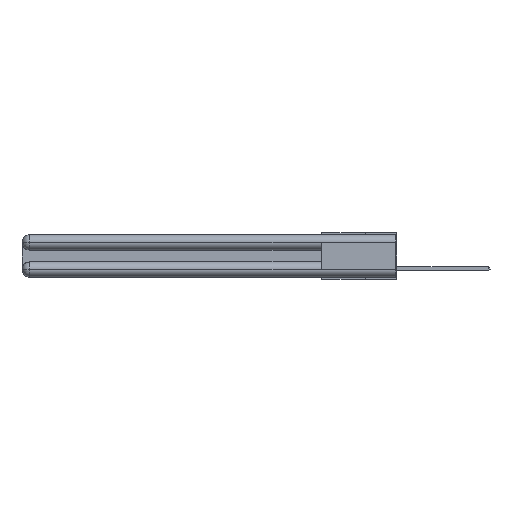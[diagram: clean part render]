
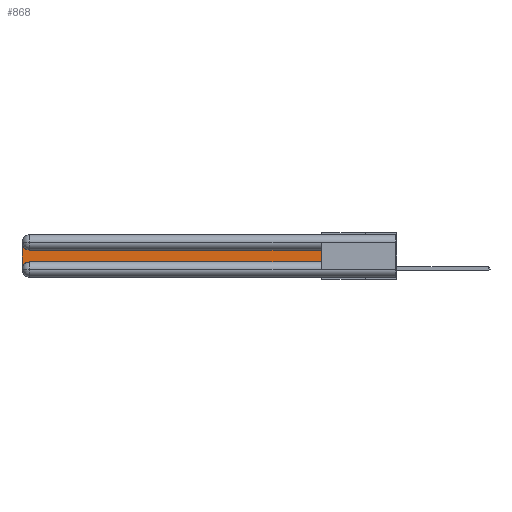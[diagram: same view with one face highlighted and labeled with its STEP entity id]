
A CAD part, left-side view. The second image highlights one B-rep face of the part: STEP entity #868.
In plain terms, the highlighted planar face has unit normal (-1, 0, 0).
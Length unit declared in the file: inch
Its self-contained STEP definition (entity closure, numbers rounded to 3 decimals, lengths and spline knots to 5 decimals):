
#131 = EDGE_CURVE ( 'NONE', #12326, #11056, #25993, .T. ) ;
#260 = PLANE ( 'NONE',  #14001 ) ;
#305 = DIRECTION ( 'NONE',  ( 1., 0., 0. ) ) ;
#825 = EDGE_CURVE ( 'NONE', #18323, #15972, #5601, .T. ) ;
#868 = ADVANCED_FACE ( 'NONE', ( #21508 ), #260, .F. ) ;
#1314 = CARTESIAN_POINT ( 'NONE',  ( 0.075, 3., -0.2175 ) ) ;
#3848 = ORIENTED_EDGE ( 'NONE', *, *, #825, .T. ) ;
#4190 = LINE ( 'NONE', #9751, #19255 ) ;
#5068 = LINE ( 'NONE', #8407, #24976 ) ;
#5601 = CIRCLE ( 'NONE', #16612, 0.06 ) ;
#8343 = LINE ( 'NONE', #31361, #13240 ) ;
#8407 = CARTESIAN_POINT ( 'NONE',  ( 0.075, 0.6, -0.2175 ) ) ;
#8570 = ORIENTED_EDGE ( 'NONE', *, *, #18665, .T. ) ;
#9751 = CARTESIAN_POINT ( 'NONE',  ( 0.075, 0.6, -0.2175 ) ) ;
#9907 = VECTOR ( 'NONE', #11904, 39.37008 ) ;
#10162 = DIRECTION ( 'NONE',  ( 0., 0., -1. ) ) ;
#11056 = VERTEX_POINT ( 'NONE', #21473 ) ;
#11326 = CARTESIAN_POINT ( 'NONE',  ( 0.075, 2.94, -0.0625 ) ) ;
#11582 = VERTEX_POINT ( 'NONE', #12493 ) ;
#11904 = DIRECTION ( 'NONE',  ( 0., 0., -1. ) ) ;
#12326 = VERTEX_POINT ( 'NONE', #15776 ) ;
#12493 = CARTESIAN_POINT ( 'NONE',  ( 0.075, 0.6, -0.2175 ) ) ;
#13110 = DIRECTION ( 'NONE',  ( 0., 0., -1. ) ) ;
#13240 = VECTOR ( 'NONE', #31790, 39.37008 ) ;
#14001 = AXIS2_PLACEMENT_3D ( 'NONE', #25837, #17995, #10162 ) ;
#14027 = EDGE_CURVE ( 'NONE', #15972, #11582, #5068, .T. ) ;
#14128 = ORIENTED_EDGE ( 'NONE', *, *, #131, .T. ) ;
#14691 = ORIENTED_EDGE ( 'NONE', *, *, #17780, .T. ) ;
#15776 = CARTESIAN_POINT ( 'NONE',  ( 0.075, 2.94, -0.1225 ) ) ;
#15972 = VERTEX_POINT ( 'NONE', #23354 ) ;
#16612 = AXIS2_PLACEMENT_3D ( 'NONE', #26168, #28786, #13110 ) ;
#17714 = AXIS2_PLACEMENT_3D ( 'NONE', #11326, #305, #21908 ) ;
#17780 = EDGE_CURVE ( 'NONE', #21364, #12326, #8343, .T. ) ;
#17995 = DIRECTION ( 'NONE',  ( 1., 0., 0. ) ) ;
#18323 = VERTEX_POINT ( 'NONE', #19178 ) ;
#18511 = EDGE_CURVE ( 'NONE', #11056, #18323, #33123, .T. ) ;
#18665 = EDGE_CURVE ( 'NONE', #11582, #21364, #4190, .T. ) ;
#18709 = CARTESIAN_POINT ( 'NONE',  ( 0.075, 0.6, -0.1225 ) ) ;
#19178 = CARTESIAN_POINT ( 'NONE',  ( 0.075, 3., -0.2775 ) ) ;
#19255 = VECTOR ( 'NONE', #31224, 39.37008 ) ;
#19655 = DIRECTION ( 'NONE',  ( 0., -1., 0. ) ) ;
#21364 = VERTEX_POINT ( 'NONE', #18709 ) ;
#21473 = CARTESIAN_POINT ( 'NONE',  ( 0.075, 3., -0.0625 ) ) ;
#21508 = FACE_OUTER_BOUND ( 'NONE', #28724, .T. ) ;
#21908 = DIRECTION ( 'NONE',  ( 0., 0., -1. ) ) ;
#22385 = ORIENTED_EDGE ( 'NONE', *, *, #14027, .T. ) ;
#23354 = CARTESIAN_POINT ( 'NONE',  ( 0.075, 2.94, -0.2175 ) ) ;
#24976 = VECTOR ( 'NONE', #19655, 39.37008 ) ;
#25837 = CARTESIAN_POINT ( 'NONE',  ( 0.075, 3., -0.1225 ) ) ;
#25993 = CIRCLE ( 'NONE', #17714, 0.06 ) ;
#26168 = CARTESIAN_POINT ( 'NONE',  ( 0.075, 2.94, -0.2775 ) ) ;
#28724 = EDGE_LOOP ( 'NONE', ( #14691, #14128, #33562, #3848, #22385, #8570 ) ) ;
#28786 = DIRECTION ( 'NONE',  ( 1., 0., 0. ) ) ;
#31224 = DIRECTION ( 'NONE',  ( 0., 0., 1. ) ) ;
#31361 = CARTESIAN_POINT ( 'NONE',  ( 0.075, 0.6, -0.1225 ) ) ;
#31790 = DIRECTION ( 'NONE',  ( 0., 1., 0. ) ) ;
#33123 = LINE ( 'NONE', #1314, #9907 ) ;
#33562 = ORIENTED_EDGE ( 'NONE', *, *, #18511, .T. ) ;
